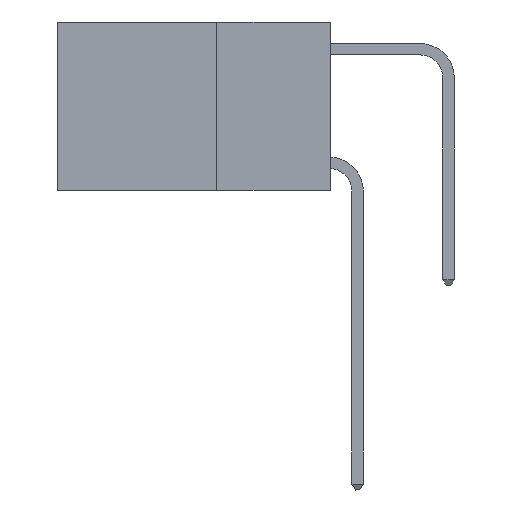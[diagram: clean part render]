
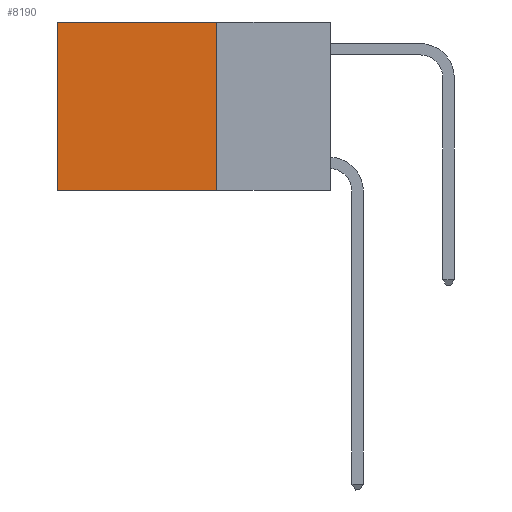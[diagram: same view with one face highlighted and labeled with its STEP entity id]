
A CAD part, left-side view. The second image highlights one B-rep face of the part: STEP entity #8190.
In plain terms, the highlighted planar face has unit normal (-1, 0, 0).
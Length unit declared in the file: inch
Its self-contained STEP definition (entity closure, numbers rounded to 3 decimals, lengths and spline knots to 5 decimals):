
#485 = EDGE_CURVE ( 'NONE', #3128, #14299, #29457, .T. ) ;
#718 = LINE ( 'NONE', #876, #13274 ) ;
#876 = CARTESIAN_POINT ( 'NONE',  ( 0.2625, 0.25, 0. ) ) ;
#1343 = EDGE_CURVE ( 'NONE', #2883, #28511, #31028, .T. ) ;
#1580 = FACE_OUTER_BOUND ( 'NONE', #23442, .T. ) ;
#2883 = VERTEX_POINT ( 'NONE', #29388 ) ;
#3128 = VERTEX_POINT ( 'NONE', #30826 ) ;
#3417 = LINE ( 'NONE', #25446, #32152 ) ;
#3526 = VECTOR ( 'NONE', #16478, 39.37008 ) ;
#4228 = ORIENTED_EDGE ( 'NONE', *, *, #485, .T. ) ;
#6322 = EDGE_CURVE ( 'NONE', #28511, #14299, #3417, .T. ) ;
#7105 = CARTESIAN_POINT ( 'NONE',  ( 0.2625, 0.6, 0. ) ) ;
#8190 = ADVANCED_FACE ( 'NONE', ( #1580 ), #24262, .F. ) ;
#9988 = ORIENTED_EDGE ( 'NONE', *, *, #15557, .T. ) ;
#10844 = DIRECTION ( 'NONE',  ( 0., 1., 0. ) ) ;
#11947 = ORIENTED_EDGE ( 'NONE', *, *, #6322, .F. ) ;
#13274 = VECTOR ( 'NONE', #10844, 39.37008 ) ;
#14299 = VERTEX_POINT ( 'NONE', #16217 ) ;
#15557 = EDGE_CURVE ( 'NONE', #2883, #3128, #718, .T. ) ;
#16217 = CARTESIAN_POINT ( 'NONE',  ( 0.2625, 0.6, -0.37 ) ) ;
#16478 = DIRECTION ( 'NONE',  ( 0., 0., -1. ) ) ;
#19296 = ORIENTED_EDGE ( 'NONE', *, *, #1343, .F. ) ;
#21645 = DIRECTION ( 'NONE',  ( 1., 0., 0. ) ) ;
#21777 = DIRECTION ( 'NONE',  ( 0., 0., -1. ) ) ;
#22847 = DIRECTION ( 'NONE',  ( 0., 1., 0. ) ) ;
#23135 = CARTESIAN_POINT ( 'NONE',  ( 0.2625, 0.25, -0.37 ) ) ;
#23442 = EDGE_LOOP ( 'NONE', ( #4228, #11947, #19296, #9988 ) ) ;
#23617 = CARTESIAN_POINT ( 'NONE',  ( 0.2625, 0.25, 0. ) ) ;
#24262 = PLANE ( 'NONE',  #30527 ) ;
#25446 = CARTESIAN_POINT ( 'NONE',  ( 0.2625, 0.25, -0.37 ) ) ;
#27926 = CARTESIAN_POINT ( 'NONE',  ( 0.2625, 0.25, 0. ) ) ;
#28511 = VERTEX_POINT ( 'NONE', #23135 ) ;
#28850 = DIRECTION ( 'NONE',  ( 0., 0., -1. ) ) ;
#29388 = CARTESIAN_POINT ( 'NONE',  ( 0.2625, 0.25, 0. ) ) ;
#29457 = LINE ( 'NONE', #7105, #30563 ) ;
#30527 = AXIS2_PLACEMENT_3D ( 'NONE', #23617, #21645, #28850 ) ;
#30563 = VECTOR ( 'NONE', #21777, 39.37008 ) ;
#30826 = CARTESIAN_POINT ( 'NONE',  ( 0.2625, 0.6, 0. ) ) ;
#31028 = LINE ( 'NONE', #27926, #3526 ) ;
#32152 = VECTOR ( 'NONE', #22847, 39.37008 ) ;
